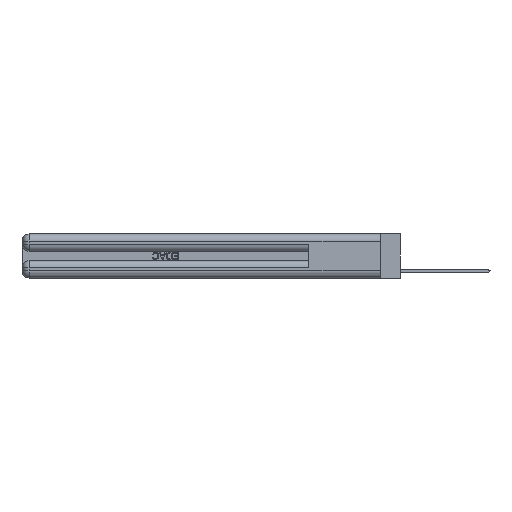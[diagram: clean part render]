
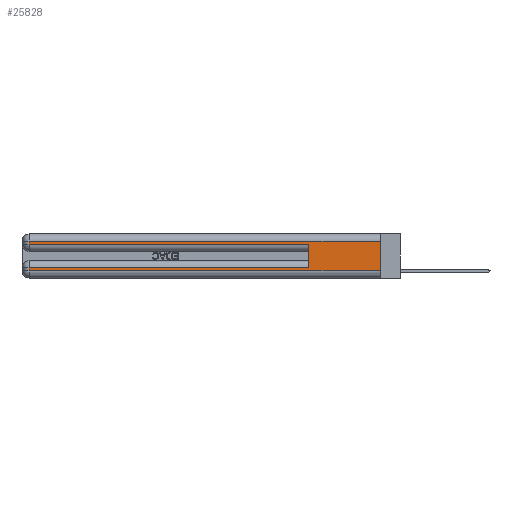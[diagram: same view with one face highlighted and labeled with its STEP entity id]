
A CAD part, left-side view. The second image highlights one B-rep face of the part: STEP entity #25828.
In plain terms, the highlighted planar face has unit normal (-1, 0, 0).
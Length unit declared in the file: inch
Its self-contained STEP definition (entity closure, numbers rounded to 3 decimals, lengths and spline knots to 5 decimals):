
#141 = VECTOR ( 'NONE', #24306, 39.37008 ) ;
#225 = EDGE_LOOP ( 'NONE', ( #20118, #13810, #20968, #17538, #1255, #9577, #22528, #31037 ) ) ;
#560 = AXIS2_PLACEMENT_3D ( 'NONE', #32434, #22235, #11499 ) ;
#1255 = ORIENTED_EDGE ( 'NONE', *, *, #17090, .F. ) ;
#2872 = CARTESIAN_POINT ( 'NONE',  ( 0., 2.94, 0.31 ) ) ;
#3169 = CARTESIAN_POINT ( 'NONE',  ( 0., 2.94, 0.37 ) ) ;
#3337 = LINE ( 'NONE', #11664, #14043 ) ;
#3485 = CARTESIAN_POINT ( 'NONE',  ( 0., 0.6, 0.085 ) ) ;
#4304 = CARTESIAN_POINT ( 'NONE',  ( 0., 2.94, 0.37 ) ) ;
#4335 = EDGE_CURVE ( 'NONE', #28314, #9807, #3337, .T. ) ;
#4337 = LINE ( 'NONE', #14885, #28721 ) ;
#4406 = EDGE_CURVE ( 'NONE', #13391, #26854, #11327, .T. ) ;
#6123 = CARTESIAN_POINT ( 'NONE',  ( 0., 0., 0.31 ) ) ;
#7178 = CARTESIAN_POINT ( 'NONE',  ( 0., 2.94, 0.06 ) ) ;
#7773 = VECTOR ( 'NONE', #32357, 39.37008 ) ;
#9346 = EDGE_CURVE ( 'NONE', #30976, #11893, #4337, .T. ) ;
#9577 = ORIENTED_EDGE ( 'NONE', *, *, #20481, .T. ) ;
#9807 = VERTEX_POINT ( 'NONE', #2872 ) ;
#11327 = LINE ( 'NONE', #3169, #141 ) ;
#11394 = CARTESIAN_POINT ( 'NONE',  ( 0., 0.6, 0.145 ) ) ;
#11499 = DIRECTION ( 'NONE',  ( 0., 0., -1. ) ) ;
#11664 = CARTESIAN_POINT ( 'NONE',  ( 0., 0., 0.31 ) ) ;
#11764 = CARTESIAN_POINT ( 'NONE',  ( 0., 0., 0.37 ) ) ;
#11893 = VERTEX_POINT ( 'NONE', #32494 ) ;
#11906 = VECTOR ( 'NONE', #33882, 39.37008 ) ;
#13391 = VERTEX_POINT ( 'NONE', #13620 ) ;
#13464 = VECTOR ( 'NONE', #17486, 39.37008 ) ;
#13620 = CARTESIAN_POINT ( 'NONE',  ( 0., 2.94, 0.085 ) ) ;
#13810 = ORIENTED_EDGE ( 'NONE', *, *, #4335, .T. ) ;
#14043 = VECTOR ( 'NONE', #32938, 39.37008 ) ;
#14273 = PLANE ( 'NONE',  #560 ) ;
#14364 = LINE ( 'NONE', #11764, #7773 ) ;
#14885 = CARTESIAN_POINT ( 'NONE',  ( 0., 0., 0.285 ) ) ;
#16723 = EDGE_CURVE ( 'NONE', #9807, #30976, #22823, .T. ) ;
#17090 = EDGE_CURVE ( 'NONE', #31807, #11893, #30067, .T. ) ;
#17486 = DIRECTION ( 'NONE',  ( 0., 1., 0. ) ) ;
#17538 = ORIENTED_EDGE ( 'NONE', *, *, #9346, .T. ) ;
#19343 = CARTESIAN_POINT ( 'NONE',  ( 0., 2.94, 0.285 ) ) ;
#19348 = DIRECTION ( 'NONE',  ( 0., 0., 1. ) ) ;
#19524 = VECTOR ( 'NONE', #20071, 39.37008 ) ;
#19688 = EDGE_CURVE ( 'NONE', #26854, #33896, #22661, .T. ) ;
#20071 = DIRECTION ( 'NONE',  ( 0., -1., 0. ) ) ;
#20118 = ORIENTED_EDGE ( 'NONE', *, *, #26324, .F. ) ;
#20481 = EDGE_CURVE ( 'NONE', #31807, #13391, #33261, .T. ) ;
#20968 = ORIENTED_EDGE ( 'NONE', *, *, #16723, .T. ) ;
#22235 = DIRECTION ( 'NONE',  ( 1., 0., 0. ) ) ;
#22528 = ORIENTED_EDGE ( 'NONE', *, *, #4406, .T. ) ;
#22661 = LINE ( 'NONE', #33214, #19524 ) ;
#22823 = LINE ( 'NONE', #4304, #11906 ) ;
#22857 = VECTOR ( 'NONE', #19348, 39.37008 ) ;
#24306 = DIRECTION ( 'NONE',  ( 0., 0., -1. ) ) ;
#25450 = DIRECTION ( 'NONE',  ( 0., -1., 0. ) ) ;
#25828 = ADVANCED_FACE ( 'NONE', ( #30337 ), #14273, .F. ) ;
#26324 = EDGE_CURVE ( 'NONE', #28314, #33896, #14364, .T. ) ;
#26854 = VERTEX_POINT ( 'NONE', #7178 ) ;
#27651 = CARTESIAN_POINT ( 'NONE',  ( 0., 0., 0.06 ) ) ;
#28314 = VERTEX_POINT ( 'NONE', #6123 ) ;
#28721 = VECTOR ( 'NONE', #25450, 39.37008 ) ;
#30067 = LINE ( 'NONE', #11394, #22857 ) ;
#30337 = FACE_OUTER_BOUND ( 'NONE', #225, .T. ) ;
#30976 = VERTEX_POINT ( 'NONE', #19343 ) ;
#31037 = ORIENTED_EDGE ( 'NONE', *, *, #19688, .T. ) ;
#31807 = VERTEX_POINT ( 'NONE', #3485 ) ;
#32357 = DIRECTION ( 'NONE',  ( 0., 0., -1. ) ) ;
#32434 = CARTESIAN_POINT ( 'NONE',  ( 0., 0., 0.37 ) ) ;
#32494 = CARTESIAN_POINT ( 'NONE',  ( 0., 0.6, 0.285 ) ) ;
#32757 = CARTESIAN_POINT ( 'NONE',  ( 0., 0., 0.085 ) ) ;
#32938 = DIRECTION ( 'NONE',  ( 0., 1., 0. ) ) ;
#33214 = CARTESIAN_POINT ( 'NONE',  ( 0., 0., 0.06 ) ) ;
#33261 = LINE ( 'NONE', #32757, #13464 ) ;
#33882 = DIRECTION ( 'NONE',  ( 0., 0., -1. ) ) ;
#33896 = VERTEX_POINT ( 'NONE', #27651 ) ;
